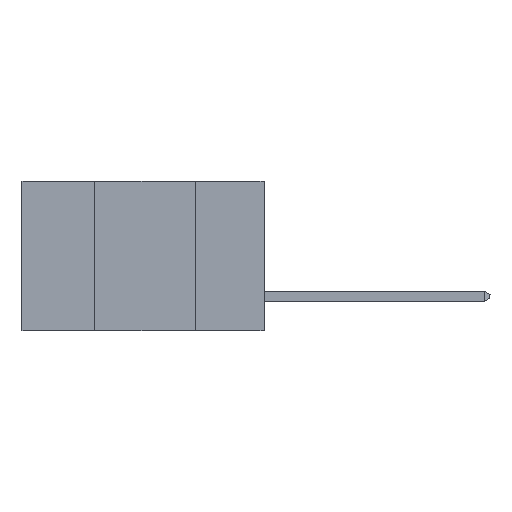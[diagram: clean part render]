
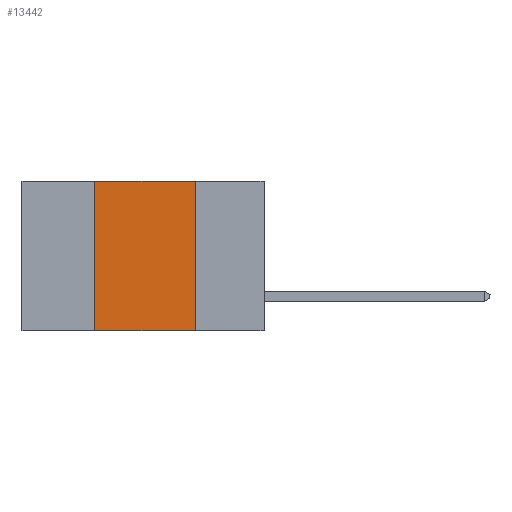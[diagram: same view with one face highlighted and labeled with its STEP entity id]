
A CAD part, left-side view. The second image highlights one B-rep face of the part: STEP entity #13442.
In plain terms, the highlighted planar face has unit normal (-1, 0, 0).
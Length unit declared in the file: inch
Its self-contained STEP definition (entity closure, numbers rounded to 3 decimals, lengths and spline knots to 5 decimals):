
#292 = EDGE_CURVE ( 'NONE', #5291, #5989, #13735, .T. ) ;
#1141 = FACE_OUTER_BOUND ( 'NONE', #10075, .T. ) ;
#2031 = EDGE_CURVE ( 'NONE', #5291, #20906, #14925, .T. ) ;
#2808 = CARTESIAN_POINT ( 'NONE',  ( 0., 0.42, 0. ) ) ;
#3459 = VECTOR ( 'NONE', #16330, 39.37008 ) ;
#3471 = VECTOR ( 'NONE', #5067, 39.37008 ) ;
#4583 = PLANE ( 'NONE',  #12278 ) ;
#5067 = DIRECTION ( 'NONE',  ( 0., -1., 0. ) ) ;
#5220 = ORIENTED_EDGE ( 'NONE', *, *, #2031, .F. ) ;
#5291 = VERTEX_POINT ( 'NONE', #7346 ) ;
#5989 = VERTEX_POINT ( 'NONE', #18470 ) ;
#6225 = DIRECTION ( 'NONE',  ( 1., 0., 0. ) ) ;
#6794 = CARTESIAN_POINT ( 'NONE',  ( 0., 0.17, 0. ) ) ;
#6942 = CARTESIAN_POINT ( 'NONE',  ( 0., 0.6, 0. ) ) ;
#7346 = CARTESIAN_POINT ( 'NONE',  ( 0., 0.42, -0.37 ) ) ;
#7766 = EDGE_CURVE ( 'NONE', #20906, #13173, #10363, .T. ) ;
#7995 = CARTESIAN_POINT ( 'NONE',  ( 0., 0.17, -0.37 ) ) ;
#10075 = EDGE_LOOP ( 'NONE', ( #11630, #14052, #5220, #21314 ) ) ;
#10249 = EDGE_CURVE ( 'NONE', #13173, #5989, #19943, .T. ) ;
#10363 = LINE ( 'NONE', #6942, #3471 ) ;
#10365 = DIRECTION ( 'NONE',  ( 0., -1., 0. ) ) ;
#11630 = ORIENTED_EDGE ( 'NONE', *, *, #10249, .F. ) ;
#12278 = AXIS2_PLACEMENT_3D ( 'NONE', #19608, #6225, #15987 ) ;
#13173 = VERTEX_POINT ( 'NONE', #6794 ) ;
#13442 = ADVANCED_FACE ( 'NONE', ( #1141 ), #4583, .F. ) ;
#13735 = LINE ( 'NONE', #18349, #21580 ) ;
#14052 = ORIENTED_EDGE ( 'NONE', *, *, #7766, .F. ) ;
#14713 = DIRECTION ( 'NONE',  ( 0., 0., 1. ) ) ;
#14925 = LINE ( 'NONE', #16582, #16756 ) ;
#15987 = DIRECTION ( 'NONE',  ( 0., 0., -1. ) ) ;
#16330 = DIRECTION ( 'NONE',  ( 0., 0., -1. ) ) ;
#16582 = CARTESIAN_POINT ( 'NONE',  ( 0., 0.42, -0.37 ) ) ;
#16756 = VECTOR ( 'NONE', #14713, 39.37008 ) ;
#18349 = CARTESIAN_POINT ( 'NONE',  ( 0., 0.6, -0.37 ) ) ;
#18470 = CARTESIAN_POINT ( 'NONE',  ( 0., 0.17, -0.37 ) ) ;
#19608 = CARTESIAN_POINT ( 'NONE',  ( 0., 0.6, 0. ) ) ;
#19943 = LINE ( 'NONE', #7995, #3459 ) ;
#20906 = VERTEX_POINT ( 'NONE', #2808 ) ;
#21314 = ORIENTED_EDGE ( 'NONE', *, *, #292, .T. ) ;
#21580 = VECTOR ( 'NONE', #10365, 39.37008 ) ;
